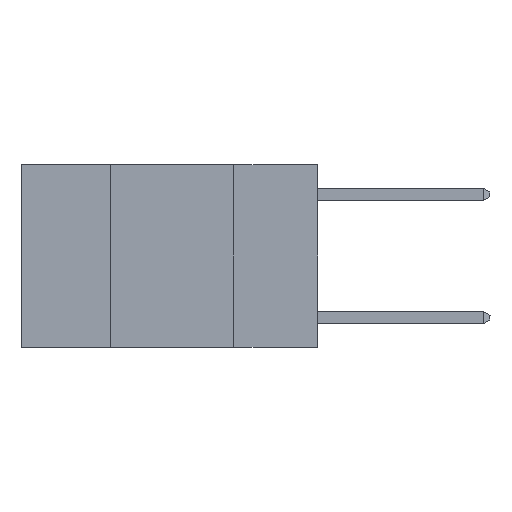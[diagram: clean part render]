
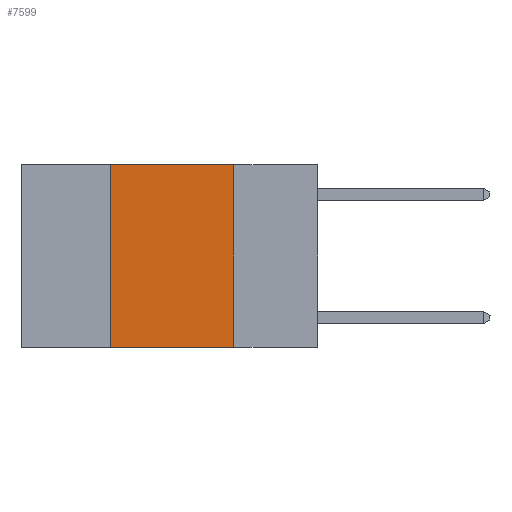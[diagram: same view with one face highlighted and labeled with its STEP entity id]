
A CAD part, left-side view. The second image highlights one B-rep face of the part: STEP entity #7599.
In plain terms, the highlighted planar face has unit normal (-1, 0, 0).
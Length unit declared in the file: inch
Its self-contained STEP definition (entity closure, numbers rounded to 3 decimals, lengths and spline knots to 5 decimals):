
#735 = CARTESIAN_POINT ( 'NONE',  ( 0., 0.42, -0.37 ) ) ;
#1197 = VECTOR ( 'NONE', #20650, 39.37008 ) ;
#1392 = LINE ( 'NONE', #15529, #5805 ) ;
#1763 = EDGE_CURVE ( 'NONE', #5163, #17899, #1392, .T. ) ;
#2745 = CARTESIAN_POINT ( 'NONE',  ( 0., 0.17, -0.37 ) ) ;
#2990 = VERTEX_POINT ( 'NONE', #10228 ) ;
#3664 = CARTESIAN_POINT ( 'NONE',  ( 0., 0.6, 0. ) ) ;
#4429 = CARTESIAN_POINT ( 'NONE',  ( 0., 0.6, 0. ) ) ;
#5163 = VERTEX_POINT ( 'NONE', #735 ) ;
#5805 = VECTOR ( 'NONE', #17126, 39.37008 ) ;
#6639 = EDGE_CURVE ( 'NONE', #5163, #2990, #14283, .T. ) ;
#6671 = VERTEX_POINT ( 'NONE', #12891 ) ;
#6955 = DIRECTION ( 'NONE',  ( 1., 0., 0. ) ) ;
#7532 = EDGE_LOOP ( 'NONE', ( #16593, #20679, #8509, #17079 ) ) ;
#7599 = ADVANCED_FACE ( 'NONE', ( #14000 ), #11695, .F. ) ;
#7945 = CARTESIAN_POINT ( 'NONE',  ( 0., 0.17, 0. ) ) ;
#8388 = LINE ( 'NONE', #4429, #11700 ) ;
#8509 = ORIENTED_EDGE ( 'NONE', *, *, #6639, .F. ) ;
#10228 = CARTESIAN_POINT ( 'NONE',  ( 0., 0.42, 0. ) ) ;
#11171 = DIRECTION ( 'NONE',  ( 0., 0., 1. ) ) ;
#11695 = PLANE ( 'NONE',  #16123 ) ;
#11700 = VECTOR ( 'NONE', #17347, 39.37008 ) ;
#12891 = CARTESIAN_POINT ( 'NONE',  ( 0., 0.17, 0. ) ) ;
#14000 = FACE_OUTER_BOUND ( 'NONE', #7532, .T. ) ;
#14283 = LINE ( 'NONE', #17527, #17980 ) ;
#15529 = CARTESIAN_POINT ( 'NONE',  ( 0., 0.6, -0.37 ) ) ;
#16123 = AXIS2_PLACEMENT_3D ( 'NONE', #3664, #6955, #18190 ) ;
#16593 = ORIENTED_EDGE ( 'NONE', *, *, #18668, .F. ) ;
#17079 = ORIENTED_EDGE ( 'NONE', *, *, #1763, .T. ) ;
#17126 = DIRECTION ( 'NONE',  ( 0., -1., 0. ) ) ;
#17347 = DIRECTION ( 'NONE',  ( 0., -1., 0. ) ) ;
#17527 = CARTESIAN_POINT ( 'NONE',  ( 0., 0.42, 0. ) ) ;
#17899 = VERTEX_POINT ( 'NONE', #2745 ) ;
#17980 = VECTOR ( 'NONE', #11171, 39.37008 ) ;
#18190 = DIRECTION ( 'NONE',  ( 0., 0., -1. ) ) ;
#18458 = LINE ( 'NONE', #7945, #1197 ) ;
#18668 = EDGE_CURVE ( 'NONE', #6671, #17899, #18458, .T. ) ;
#19255 = EDGE_CURVE ( 'NONE', #2990, #6671, #8388, .T. ) ;
#20650 = DIRECTION ( 'NONE',  ( 0., 0., -1. ) ) ;
#20679 = ORIENTED_EDGE ( 'NONE', *, *, #19255, .F. ) ;
